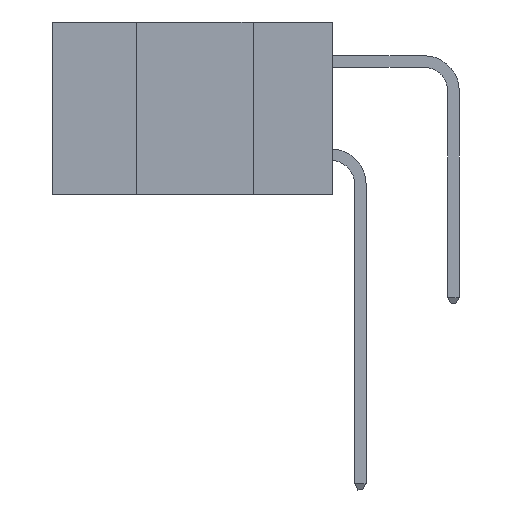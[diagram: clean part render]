
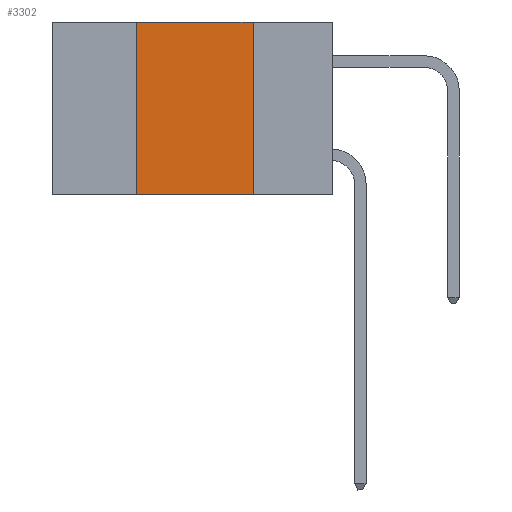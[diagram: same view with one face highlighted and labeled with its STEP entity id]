
A CAD part, left-side view. The second image highlights one B-rep face of the part: STEP entity #3302.
In plain terms, the highlighted planar face has unit normal (-1, 0, 0).
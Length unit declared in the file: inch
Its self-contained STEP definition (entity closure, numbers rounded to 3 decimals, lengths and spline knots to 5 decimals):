
#56 = DIRECTION ( 'NONE',  ( 0., 0., 1. ) ) ;
#211 = LINE ( 'NONE', #12083, #28067 ) ;
#702 = CARTESIAN_POINT ( 'NONE',  ( 0., 0.6, -0.37 ) ) ;
#869 = DIRECTION ( 'NONE',  ( 0., -1., 0. ) ) ;
#1341 = VERTEX_POINT ( 'NONE', #2499 ) ;
#2499 = CARTESIAN_POINT ( 'NONE',  ( 0., 0.42, -0.37 ) ) ;
#3302 = ADVANCED_FACE ( 'NONE', ( #8383 ), #21206, .F. ) ;
#3508 = DIRECTION ( 'NONE',  ( 0., 0., -1. ) ) ;
#3940 = VERTEX_POINT ( 'NONE', #20266 ) ;
#4240 = AXIS2_PLACEMENT_3D ( 'NONE', #22365, #25828, #25796 ) ;
#5446 = EDGE_CURVE ( 'NONE', #11607, #3940, #12109, .T. ) ;
#5496 = VECTOR ( 'NONE', #3508, 39.37008 ) ;
#6595 = VERTEX_POINT ( 'NONE', #16826 ) ;
#8383 = FACE_OUTER_BOUND ( 'NONE', #14550, .T. ) ;
#9540 = VECTOR ( 'NONE', #56, 39.37008 ) ;
#9923 = CARTESIAN_POINT ( 'NONE',  ( 0., 0.17, 0. ) ) ;
#11607 = VERTEX_POINT ( 'NONE', #9923 ) ;
#11917 = LINE ( 'NONE', #702, #17715 ) ;
#11924 = DIRECTION ( 'NONE',  ( 0., -1., 0. ) ) ;
#12083 = CARTESIAN_POINT ( 'NONE',  ( 0., 0.6, 0. ) ) ;
#12109 = LINE ( 'NONE', #24705, #5496 ) ;
#13013 = EDGE_CURVE ( 'NONE', #1341, #3940, #11917, .T. ) ;
#14550 = EDGE_LOOP ( 'NONE', ( #16041, #27292, #22484, #23638 ) ) ;
#14664 = LINE ( 'NONE', #15693, #9540 ) ;
#15693 = CARTESIAN_POINT ( 'NONE',  ( 0., 0.42, -0.37 ) ) ;
#16041 = ORIENTED_EDGE ( 'NONE', *, *, #5446, .F. ) ;
#16826 = CARTESIAN_POINT ( 'NONE',  ( 0., 0.42, 0. ) ) ;
#17715 = VECTOR ( 'NONE', #11924, 39.37008 ) ;
#18888 = EDGE_CURVE ( 'NONE', #6595, #11607, #211, .T. ) ;
#20266 = CARTESIAN_POINT ( 'NONE',  ( 0., 0.17, -0.37 ) ) ;
#21206 = PLANE ( 'NONE',  #4240 ) ;
#22365 = CARTESIAN_POINT ( 'NONE',  ( 0., 0.6, 0. ) ) ;
#22484 = ORIENTED_EDGE ( 'NONE', *, *, #27509, .F. ) ;
#23638 = ORIENTED_EDGE ( 'NONE', *, *, #13013, .T. ) ;
#24705 = CARTESIAN_POINT ( 'NONE',  ( 0., 0.17, -0.37 ) ) ;
#25796 = DIRECTION ( 'NONE',  ( 0., 0., -1. ) ) ;
#25828 = DIRECTION ( 'NONE',  ( 1., 0., 0. ) ) ;
#27292 = ORIENTED_EDGE ( 'NONE', *, *, #18888, .F. ) ;
#27509 = EDGE_CURVE ( 'NONE', #1341, #6595, #14664, .T. ) ;
#28067 = VECTOR ( 'NONE', #869, 39.37008 ) ;
